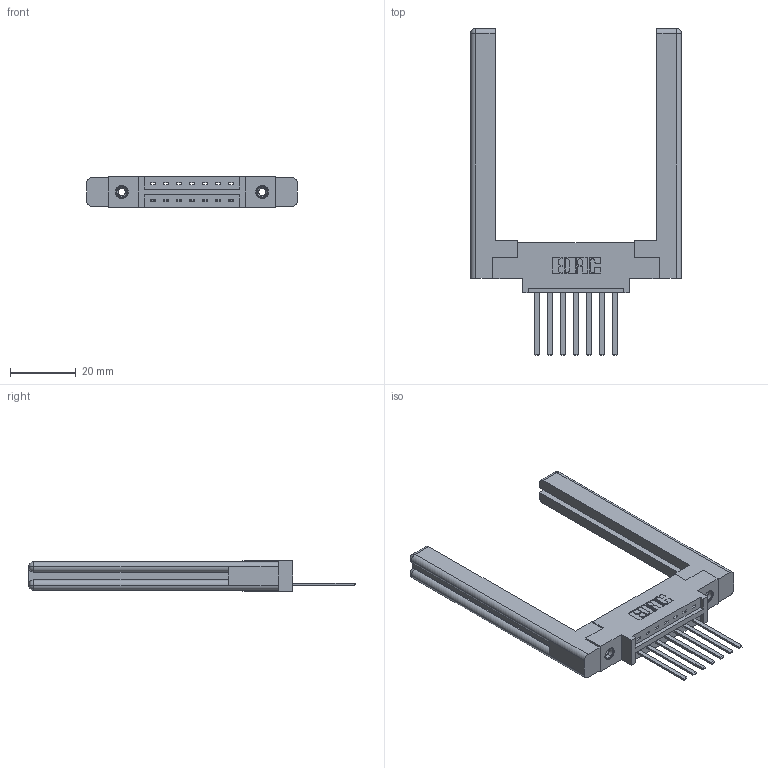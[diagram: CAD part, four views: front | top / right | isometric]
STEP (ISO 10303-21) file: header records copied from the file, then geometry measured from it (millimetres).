
FILE_DESCRIPTION (( 'STEP AP203' ), '1' );
FILE_NAME ('337-007-544-658.STEP', '2019-09-27T18:20:57', ( '' ), ( '' ), 'SwSTEP 2.0', 'SolidWorks 2016', '' );
FILE_SCHEMA (( 'CONFIG_CONTROL_DESIGN' ));
Length unit declared in the file: inch
Products named in the file (5): 345-250-001_345-250-001-102; 345-292-001_345-293-144; 307-220-058; 337-007-544-658; 337 Part_0.170 Offset - 0.156 Dia-TI
Assembly tree (12 placements, depth 2):
  337-007-544-658
    337 Part_0.170 Offset - 0.156 Dia-TI
    345-292-001_345-293-144  x7
    345-250-001_345-250-001-102  x2
    307-220-058  x2
Bounding box: 64.36 x 99.7 x 9.4 mm (x, y, z)
Volume: 13377.2 mm3; surface area: 11804.3 mm2
Topology: 12 solids, 12 shells, 652 faces, 1867 edges, 1222 vertices
Faces by surface type: plane 452, cylinder 176, cone 12, torus 12
Entity records: 12312 total; most frequent: CARTESIAN_POINT 2142, ORIENTED_EDGE 2024, DIRECTION 1890, EDGE_CURVE 1012, LINE 840, VECTOR 840, VERTEX_POINT 666, AXIS2_PLACEMENT_3D 525
